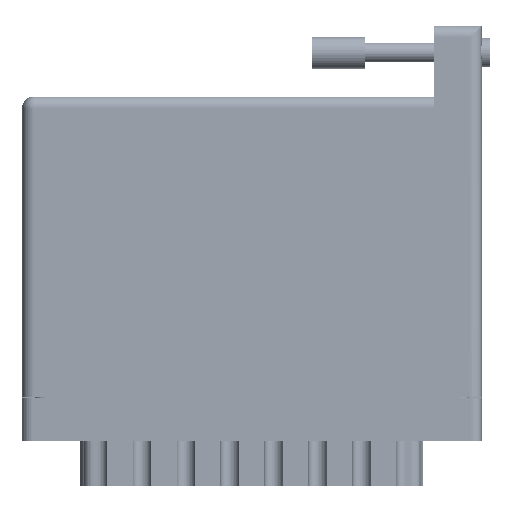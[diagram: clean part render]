
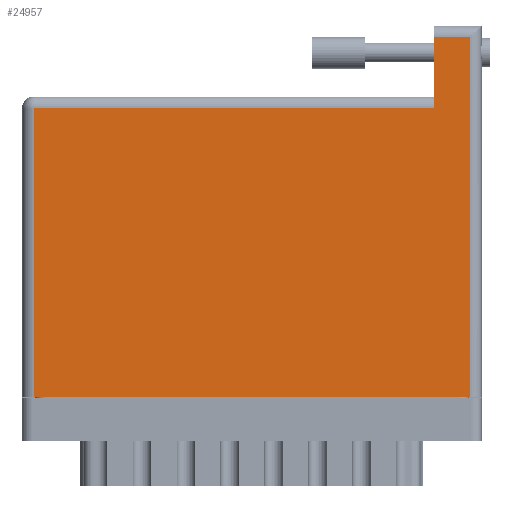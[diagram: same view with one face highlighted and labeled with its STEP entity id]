
A CAD part, front view. The second image highlights one B-rep face of the part: STEP entity #24957.
In plain terms, the highlighted face is planar.
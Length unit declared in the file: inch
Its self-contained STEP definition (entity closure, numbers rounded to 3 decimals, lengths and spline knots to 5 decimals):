
#344 = PLANE ( 'NONE',  #61867 ) ;
#2026 = DIRECTION ( 'NONE',  ( -1., 0., 0. ) ) ;
#6545 = DIRECTION ( 'NONE',  ( 0., 0., -1. ) ) ;
#8099 = CARTESIAN_POINT ( 'NONE',  ( 2.438, 2.125, 0. ) ) ;
#8180 = EDGE_CURVE ( 'NONE', #57629, #37168, #60081, .T. ) ;
#10368 = DIRECTION ( 'NONE',  ( 0., -1., 0. ) ) ;
#10736 = LINE ( 'NONE', #18245, #13575 ) ;
#13575 = VECTOR ( 'NONE', #36055, 39.37008 ) ;
#14623 = CARTESIAN_POINT ( 'NONE',  ( 2.438, 1.705, 0. ) ) ;
#15008 = VECTOR ( 'NONE', #34882, 39.37008 ) ;
#18245 = CARTESIAN_POINT ( 'NONE',  ( 0., 1.705, 0. ) ) ;
#18411 = DIRECTION ( 'NONE',  ( -1., 0., 0. ) ) ;
#20035 = DIRECTION ( 'NONE',  ( 1., 0., 0. ) ) ;
#21512 = VERTEX_POINT ( 'NONE', #32359 ) ;
#21589 = EDGE_LOOP ( 'NONE', ( #28115, #44290, #46903, #51199, #25591, #32936 ) ) ;
#24068 = CARTESIAN_POINT ( 'NONE',  ( 2.648, 2.125, 0. ) ) ;
#24957 = ADVANCED_FACE ( 'NONE', ( #52358 ), #344, .F. ) ;
#25591 = ORIENTED_EDGE ( 'NONE', *, *, #8180, .T. ) ;
#28115 = ORIENTED_EDGE ( 'NONE', *, *, #46198, .T. ) ;
#29339 = VERTEX_POINT ( 'NONE', #14623 ) ;
#30443 = EDGE_CURVE ( 'NONE', #21512, #57629, #49594, .T. ) ;
#32359 = CARTESIAN_POINT ( 'NONE',  ( 2.648, 0., 0. ) ) ;
#32936 = ORIENTED_EDGE ( 'NONE', *, *, #40927, .T. ) ;
#33257 = VERTEX_POINT ( 'NONE', #52987 ) ;
#33496 = VERTEX_POINT ( 'NONE', #50127 ) ;
#34882 = DIRECTION ( 'NONE',  ( 0., -1., 0. ) ) ;
#36055 = DIRECTION ( 'NONE',  ( -1., 0., 0. ) ) ;
#37168 = VERTEX_POINT ( 'NONE', #8099 ) ;
#40798 = VECTOR ( 'NONE', #20035, 39.37008 ) ;
#40927 = EDGE_CURVE ( 'NONE', #37168, #29339, #60299, .T. ) ;
#41410 = VECTOR ( 'NONE', #10368, 39.37008 ) ;
#42659 = LINE ( 'NONE', #49647, #40798 ) ;
#44290 = ORIENTED_EDGE ( 'NONE', *, *, #64429, .T. ) ;
#45298 = VECTOR ( 'NONE', #2026, 39.37008 ) ;
#46198 = EDGE_CURVE ( 'NONE', #29339, #33257, #10736, .T. ) ;
#46903 = ORIENTED_EDGE ( 'NONE', *, *, #61462, .T. ) ;
#47799 = CARTESIAN_POINT ( 'NONE',  ( 0., 1.775, 0. ) ) ;
#48949 = CARTESIAN_POINT ( 'NONE',  ( 0., 2.125, 0. ) ) ;
#49594 = LINE ( 'NONE', #56500, #51450 ) ;
#49647 = CARTESIAN_POINT ( 'NONE',  ( 0., 0., 0. ) ) ;
#50127 = CARTESIAN_POINT ( 'NONE',  ( 0.07, 0., 0. ) ) ;
#51199 = ORIENTED_EDGE ( 'NONE', *, *, #30443, .T. ) ;
#51450 = VECTOR ( 'NONE', #73514, 39.37008 ) ;
#51875 = CARTESIAN_POINT ( 'NONE',  ( 2.438, 2.195, 0. ) ) ;
#52358 = FACE_OUTER_BOUND ( 'NONE', #21589, .T. ) ;
#52987 = CARTESIAN_POINT ( 'NONE',  ( 0.07, 1.705, 0. ) ) ;
#56500 = CARTESIAN_POINT ( 'NONE',  ( 2.648, 2.195, 0. ) ) ;
#57629 = VERTEX_POINT ( 'NONE', #24068 ) ;
#60081 = LINE ( 'NONE', #48949, #45298 ) ;
#60299 = LINE ( 'NONE', #51875, #15008 ) ;
#61462 = EDGE_CURVE ( 'NONE', #33496, #21512, #42659, .T. ) ;
#61867 = AXIS2_PLACEMENT_3D ( 'NONE', #47799, #6545, #18411 ) ;
#63270 = CARTESIAN_POINT ( 'NONE',  ( 0.07, 0., 0. ) ) ;
#64429 = EDGE_CURVE ( 'NONE', #33257, #33496, #72744, .T. ) ;
#72744 = LINE ( 'NONE', #63270, #41410 ) ;
#73514 = DIRECTION ( 'NONE',  ( 0., 1., 0. ) ) ;
